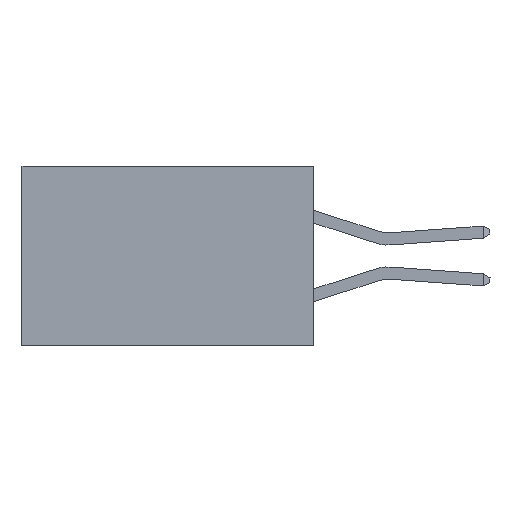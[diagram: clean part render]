
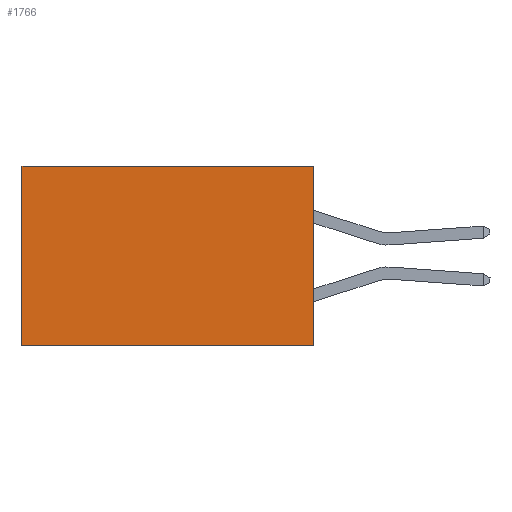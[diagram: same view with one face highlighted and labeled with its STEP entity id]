
A CAD part, left-side view. The second image highlights one B-rep face of the part: STEP entity #1766.
In plain terms, the highlighted planar face has unit normal (-1, 0, 0).
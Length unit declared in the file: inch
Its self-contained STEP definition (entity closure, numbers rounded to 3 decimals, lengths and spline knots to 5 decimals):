
#620 = FACE_OUTER_BOUND ( 'NONE', #18490, .T. ) ;
#634 = DIRECTION ( 'NONE',  ( 0., 0., -1. ) ) ;
#1443 = PLANE ( 'NONE',  #10745 ) ;
#1544 = ORIENTED_EDGE ( 'NONE', *, *, #13022, .F. ) ;
#1766 = ADVANCED_FACE ( 'NONE', ( #620 ), #1443, .F. ) ;
#1803 = VERTEX_POINT ( 'NONE', #13886 ) ;
#2190 = LINE ( 'NONE', #12620, #10764 ) ;
#4372 = CARTESIAN_POINT ( 'NONE',  ( 0.2875, 0., 0. ) ) ;
#4714 = ORIENTED_EDGE ( 'NONE', *, *, #15424, .T. ) ;
#4918 = CARTESIAN_POINT ( 'NONE',  ( 0.2875, 0.6, 0. ) ) ;
#5131 = VERTEX_POINT ( 'NONE', #6797 ) ;
#5600 = DIRECTION ( 'NONE',  ( 1., 0., 0. ) ) ;
#6024 = DIRECTION ( 'NONE',  ( 0., 1., 0. ) ) ;
#6493 = VERTEX_POINT ( 'NONE', #8823 ) ;
#6797 = CARTESIAN_POINT ( 'NONE',  ( 0.2875, 0., 0. ) ) ;
#8823 = CARTESIAN_POINT ( 'NONE',  ( 0.2875, 0.6, 0. ) ) ;
#10745 = AXIS2_PLACEMENT_3D ( 'NONE', #21251, #5600, #17495 ) ;
#10764 = VECTOR ( 'NONE', #14316, 39.37008 ) ;
#11172 = EDGE_CURVE ( 'NONE', #5131, #6493, #13712, .T. ) ;
#11504 = LINE ( 'NONE', #17771, #19567 ) ;
#12620 = CARTESIAN_POINT ( 'NONE',  ( 0.2875, 0., -0.37 ) ) ;
#12752 = LINE ( 'NONE', #4918, #21865 ) ;
#13022 = EDGE_CURVE ( 'NONE', #5131, #1803, #11504, .T. ) ;
#13712 = LINE ( 'NONE', #4372, #17760 ) ;
#13886 = CARTESIAN_POINT ( 'NONE',  ( 0.2875, 0., -0.37 ) ) ;
#14142 = ORIENTED_EDGE ( 'NONE', *, *, #18794, .F. ) ;
#14316 = DIRECTION ( 'NONE',  ( 0., 1., 0. ) ) ;
#15076 = DIRECTION ( 'NONE',  ( 0., 0., -1. ) ) ;
#15424 = EDGE_CURVE ( 'NONE', #6493, #16879, #12752, .T. ) ;
#16528 = ORIENTED_EDGE ( 'NONE', *, *, #11172, .T. ) ;
#16879 = VERTEX_POINT ( 'NONE', #17427 ) ;
#17427 = CARTESIAN_POINT ( 'NONE',  ( 0.2875, 0.6, -0.37 ) ) ;
#17495 = DIRECTION ( 'NONE',  ( 0., 0., -1. ) ) ;
#17760 = VECTOR ( 'NONE', #6024, 39.37008 ) ;
#17771 = CARTESIAN_POINT ( 'NONE',  ( 0.2875, 0., 0. ) ) ;
#18490 = EDGE_LOOP ( 'NONE', ( #4714, #14142, #1544, #16528 ) ) ;
#18794 = EDGE_CURVE ( 'NONE', #1803, #16879, #2190, .T. ) ;
#19567 = VECTOR ( 'NONE', #634, 39.37008 ) ;
#21251 = CARTESIAN_POINT ( 'NONE',  ( 0.2875, 0., 0. ) ) ;
#21865 = VECTOR ( 'NONE', #15076, 39.37008 ) ;
